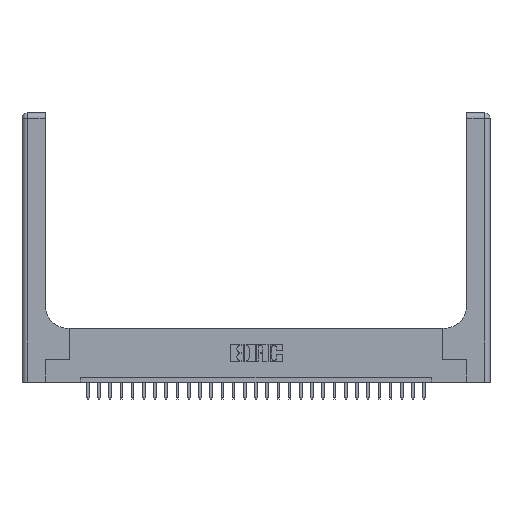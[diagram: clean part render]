
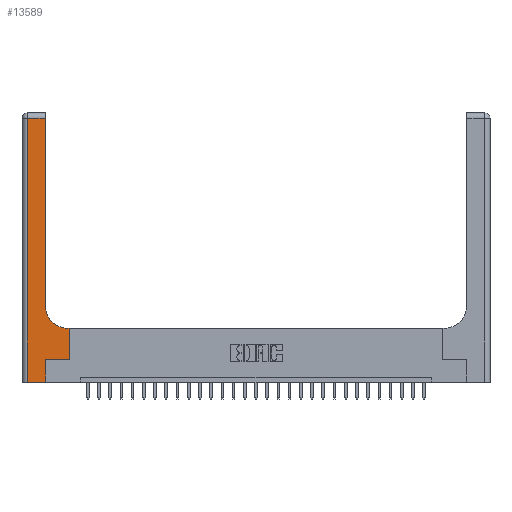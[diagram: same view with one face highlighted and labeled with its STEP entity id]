
A CAD part, top view. The second image highlights one B-rep face of the part: STEP entity #13589.
In plain terms, the highlighted planar face has unit normal (0, 0, 1).
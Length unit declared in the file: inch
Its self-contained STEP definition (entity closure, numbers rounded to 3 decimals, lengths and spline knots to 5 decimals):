
#563 = LINE ( 'NONE', #13210, #7197 ) ;
#625 = EDGE_CURVE ( 'NONE', #2163, #6441, #22717, .T. ) ;
#726 = VECTOR ( 'NONE', #7618, 39.37008 ) ;
#892 = CARTESIAN_POINT ( 'NONE',  ( 0.26, 0.85, 0.37 ) ) ;
#1686 = CARTESIAN_POINT ( 'NONE',  ( 0.265, 0.25, 0.37 ) ) ;
#2163 = VERTEX_POINT ( 'NONE', #15262 ) ;
#2856 = CARTESIAN_POINT ( 'NONE',  ( 0., 0., 0.37 ) ) ;
#2872 = EDGE_CURVE ( 'NONE', #20269, #8836, #7241, .T. ) ;
#3395 = FACE_OUTER_BOUND ( 'NONE', #9114, .T. ) ;
#3405 = DIRECTION ( 'NONE',  ( 1., 0., 0. ) ) ;
#3448 = VECTOR ( 'NONE', #23305, 39.37008 ) ;
#3512 = VECTOR ( 'NONE', #8013, 39.37008 ) ;
#4046 = ORIENTED_EDGE ( 'NONE', *, *, #625, .T. ) ;
#4318 = EDGE_CURVE ( 'NONE', #6441, #18718, #18135, .T. ) ;
#5189 = ORIENTED_EDGE ( 'NONE', *, *, #4318, .T. ) ;
#5222 = DIRECTION ( 'NONE',  ( 0., 1., 0. ) ) ;
#5610 = CARTESIAN_POINT ( 'NONE',  ( 0., 2.94, 0.37 ) ) ;
#5620 = VECTOR ( 'NONE', #9732, 39.37008 ) ;
#5991 = DIRECTION ( 'NONE',  ( 0., 1., 0. ) ) ;
#6118 = EDGE_CURVE ( 'NONE', #10028, #13415, #7936, .T. ) ;
#6441 = VERTEX_POINT ( 'NONE', #7306 ) ;
#7197 = VECTOR ( 'NONE', #5222, 39.37008 ) ;
#7241 = CIRCLE ( 'NONE', #25418, 0.25 ) ;
#7306 = CARTESIAN_POINT ( 'NONE',  ( 0.265, 0.25, 0.37 ) ) ;
#7535 = ORIENTED_EDGE ( 'NONE', *, *, #6118, .T. ) ;
#7618 = DIRECTION ( 'NONE',  ( 0., 1., 0. ) ) ;
#7702 = VERTEX_POINT ( 'NONE', #24675 ) ;
#7936 = LINE ( 'NONE', #14015, #3512 ) ;
#8013 = DIRECTION ( 'NONE',  ( 0., -1., 0. ) ) ;
#8836 = VERTEX_POINT ( 'NONE', #892 ) ;
#8911 = EDGE_CURVE ( 'NONE', #8836, #12000, #563, .T. ) ;
#9114 = EDGE_LOOP ( 'NONE', ( #17583, #19467, #7535, #26020, #4046, #5189, #17209, #12907, #25422 ) ) ;
#9316 = EDGE_CURVE ( 'NONE', #7702, #20269, #23172, .T. ) ;
#9732 = DIRECTION ( 'NONE',  ( -1., 0., 0. ) ) ;
#9799 = VECTOR ( 'NONE', #5991, 39.37008 ) ;
#9977 = PLANE ( 'NONE',  #14312 ) ;
#10028 = VERTEX_POINT ( 'NONE', #15964 ) ;
#11555 = CARTESIAN_POINT ( 'NONE',  ( 0.265, 0., 0.37 ) ) ;
#12000 = VERTEX_POINT ( 'NONE', #12039 ) ;
#12039 = CARTESIAN_POINT ( 'NONE',  ( 0.26, 2.94, 0.37 ) ) ;
#12114 = CARTESIAN_POINT ( 'NONE',  ( 0.528, 0.25, 0.37 ) ) ;
#12282 = VECTOR ( 'NONE', #23034, 39.37008 ) ;
#12674 = CARTESIAN_POINT ( 'NONE',  ( 0.06, 0., 0.37 ) ) ;
#12801 = VECTOR ( 'NONE', #17775, 39.37008 ) ;
#12907 = ORIENTED_EDGE ( 'NONE', *, *, #9316, .T. ) ;
#13210 = CARTESIAN_POINT ( 'NONE',  ( 0.26, 3., 0.37 ) ) ;
#13415 = VERTEX_POINT ( 'NONE', #12674 ) ;
#13546 = CARTESIAN_POINT ( 'NONE',  ( 0.26, 0.6, 0.37 ) ) ;
#13589 = ADVANCED_FACE ( 'NONE', ( #3395 ), #9977, .F. ) ;
#14015 = CARTESIAN_POINT ( 'NONE',  ( 0.06, 3., 0.37 ) ) ;
#14186 = CARTESIAN_POINT ( 'NONE',  ( 0.51, 0.6, 0.37 ) ) ;
#14312 = AXIS2_PLACEMENT_3D ( 'NONE', #24118, #17827, #18087 ) ;
#15262 = CARTESIAN_POINT ( 'NONE',  ( 0.265, 0., 0.37 ) ) ;
#15384 = DIRECTION ( 'NONE',  ( 0., 0., -1. ) ) ;
#15964 = CARTESIAN_POINT ( 'NONE',  ( 0.06, 2.94, 0.37 ) ) ;
#17209 = ORIENTED_EDGE ( 'NONE', *, *, #17727, .T. ) ;
#17583 = ORIENTED_EDGE ( 'NONE', *, *, #8911, .T. ) ;
#17727 = EDGE_CURVE ( 'NONE', #18718, #7702, #25506, .T. ) ;
#17775 = DIRECTION ( 'NONE',  ( 1., 0., 0. ) ) ;
#17827 = DIRECTION ( 'NONE',  ( 0., 0., -1. ) ) ;
#18087 = DIRECTION ( 'NONE',  ( -1., 0., 0. ) ) ;
#18135 = LINE ( 'NONE', #1686, #12801 ) ;
#18718 = VERTEX_POINT ( 'NONE', #19615 ) ;
#19350 = CARTESIAN_POINT ( 'NONE',  ( 0.51, 0.85, 0.37 ) ) ;
#19467 = ORIENTED_EDGE ( 'NONE', *, *, #24383, .T. ) ;
#19615 = CARTESIAN_POINT ( 'NONE',  ( 0.528, 0.25, 0.37 ) ) ;
#19820 = LINE ( 'NONE', #5610, #3448 ) ;
#20269 = VERTEX_POINT ( 'NONE', #14186 ) ;
#22717 = LINE ( 'NONE', #11555, #726 ) ;
#22958 = LINE ( 'NONE', #2856, #12282 ) ;
#23034 = DIRECTION ( 'NONE',  ( 1., 0., 0. ) ) ;
#23172 = LINE ( 'NONE', #13546, #5620 ) ;
#23305 = DIRECTION ( 'NONE',  ( -1., 0., 0. ) ) ;
#24050 = EDGE_CURVE ( 'NONE', #13415, #2163, #22958, .T. ) ;
#24118 = CARTESIAN_POINT ( 'NONE',  ( 0., 3., 0.37 ) ) ;
#24383 = EDGE_CURVE ( 'NONE', #12000, #10028, #19820, .T. ) ;
#24675 = CARTESIAN_POINT ( 'NONE',  ( 0.528, 0.6, 0.37 ) ) ;
#25418 = AXIS2_PLACEMENT_3D ( 'NONE', #19350, #15384, #3405 ) ;
#25422 = ORIENTED_EDGE ( 'NONE', *, *, #2872, .T. ) ;
#25506 = LINE ( 'NONE', #12114, #9799 ) ;
#26020 = ORIENTED_EDGE ( 'NONE', *, *, #24050, .T. ) ;
